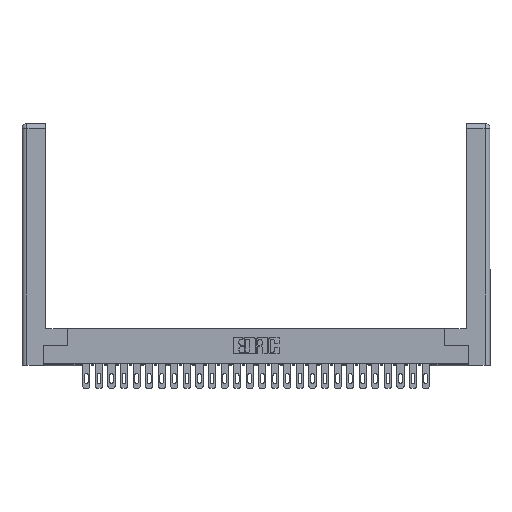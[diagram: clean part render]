
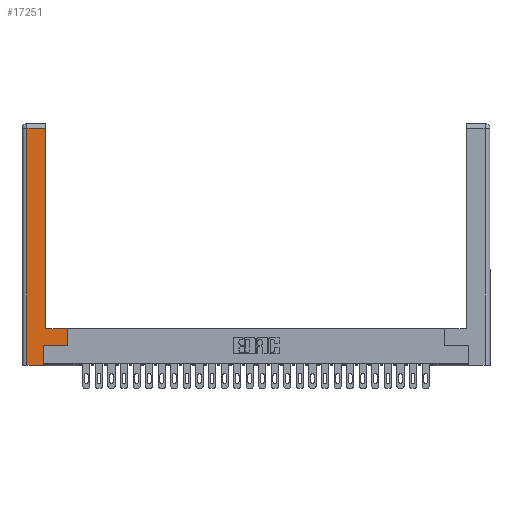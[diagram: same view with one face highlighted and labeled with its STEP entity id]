
A CAD part, top view. The second image highlights one B-rep face of the part: STEP entity #17251.
In plain terms, the highlighted planar face has unit normal (0, 0, 1).
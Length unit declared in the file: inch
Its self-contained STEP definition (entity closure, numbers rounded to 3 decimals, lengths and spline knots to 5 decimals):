
#366 = DIRECTION ( 'NONE',  ( 0., 1., 0. ) ) ;
#792 = VERTEX_POINT ( 'NONE', #11944 ) ;
#869 = LINE ( 'NONE', #4370, #18918 ) ;
#1050 = CARTESIAN_POINT ( 'NONE',  ( 0.265, 0., 0. ) ) ;
#1167 = EDGE_CURVE ( 'NONE', #3997, #29293, #11159, .T. ) ;
#1539 = VERTEX_POINT ( 'NONE', #33579 ) ;
#2278 = CARTESIAN_POINT ( 'NONE',  ( 0.0615, 0., 0. ) ) ;
#3301 = LINE ( 'NONE', #23552, #14991 ) ;
#3997 = VERTEX_POINT ( 'NONE', #1050 ) ;
#4370 = CARTESIAN_POINT ( 'NONE',  ( 0.0615, 2.94, 0. ) ) ;
#4867 = CARTESIAN_POINT ( 'NONE',  ( 0.565, 0.45, 0. ) ) ;
#5165 = VECTOR ( 'NONE', #31440, 39.37008 ) ;
#6160 = CARTESIAN_POINT ( 'NONE',  ( 0.565, 0.245, 0. ) ) ;
#6353 = ORIENTED_EDGE ( 'NONE', *, *, #8636, .T. ) ;
#6360 = VERTEX_POINT ( 'NONE', #4867 ) ;
#8636 = EDGE_CURVE ( 'NONE', #792, #27243, #3301, .T. ) ;
#8668 = EDGE_CURVE ( 'NONE', #28972, #1539, #8693, .T. ) ;
#8693 = LINE ( 'NONE', #2278, #28437 ) ;
#8758 = CARTESIAN_POINT ( 'NONE',  ( 0.265, 0., 0. ) ) ;
#8772 = ORIENTED_EDGE ( 'NONE', *, *, #8668, .T. ) ;
#8880 = DIRECTION ( 'NONE',  ( 1., 0., 0. ) ) ;
#9170 = EDGE_LOOP ( 'NONE', ( #6353, #10185, #8772, #30987, #24147, #32800, #30536, #9584 ) ) ;
#9584 = ORIENTED_EDGE ( 'NONE', *, *, #18812, .T. ) ;
#10185 = ORIENTED_EDGE ( 'NONE', *, *, #20304, .T. ) ;
#10280 = PLANE ( 'NONE',  #26566 ) ;
#10518 = CARTESIAN_POINT ( 'NONE',  ( 0., 0., 0. ) ) ;
#11159 = LINE ( 'NONE', #17291, #24632 ) ;
#11944 = CARTESIAN_POINT ( 'NONE',  ( 0.295, 0.45, 0. ) ) ;
#12806 = VERTEX_POINT ( 'NONE', #29446 ) ;
#13016 = FACE_OUTER_BOUND ( 'NONE', #9170, .T. ) ;
#13491 = VECTOR ( 'NONE', #22264, 39.37008 ) ;
#14577 = CARTESIAN_POINT ( 'NONE',  ( 0.265, 0.245, 0. ) ) ;
#14991 = VECTOR ( 'NONE', #29115, 39.37008 ) ;
#15316 = EDGE_CURVE ( 'NONE', #29293, #12806, #17344, .T. ) ;
#16538 = CARTESIAN_POINT ( 'NONE',  ( 0.295, 2.94, 0. ) ) ;
#17251 = ADVANCED_FACE ( 'NONE', ( #13016 ), #10280, .F. ) ;
#17291 = CARTESIAN_POINT ( 'NONE',  ( 0.265, 0.245, 0. ) ) ;
#17344 = LINE ( 'NONE', #6160, #23263 ) ;
#18119 = CARTESIAN_POINT ( 'NONE',  ( 0.0615, 2.94, 0. ) ) ;
#18812 = EDGE_CURVE ( 'NONE', #6360, #792, #27388, .T. ) ;
#18918 = VECTOR ( 'NONE', #33819, 39.37008 ) ;
#20125 = DIRECTION ( 'NONE',  ( 0., 1., 0. ) ) ;
#20160 = EDGE_CURVE ( 'NONE', #1539, #3997, #24446, .T. ) ;
#20304 = EDGE_CURVE ( 'NONE', #27243, #28972, #869, .T. ) ;
#20725 = CARTESIAN_POINT ( 'NONE',  ( 0.295, 0.45, 0. ) ) ;
#22264 = DIRECTION ( 'NONE',  ( 1., 0., 0. ) ) ;
#23263 = VECTOR ( 'NONE', #8880, 39.37008 ) ;
#23552 = CARTESIAN_POINT ( 'NONE',  ( 0.295, 3., 0. ) ) ;
#23780 = DIRECTION ( 'NONE',  ( 0., -1., 0. ) ) ;
#24147 = ORIENTED_EDGE ( 'NONE', *, *, #1167, .T. ) ;
#24227 = CARTESIAN_POINT ( 'NONE',  ( 0.565, 0.45, 0. ) ) ;
#24446 = LINE ( 'NONE', #8758, #13491 ) ;
#24632 = VECTOR ( 'NONE', #20125, 39.37008 ) ;
#26566 = AXIS2_PLACEMENT_3D ( 'NONE', #10518, #34619, #32057 ) ;
#27243 = VERTEX_POINT ( 'NONE', #16538 ) ;
#27388 = LINE ( 'NONE', #20725, #5165 ) ;
#28437 = VECTOR ( 'NONE', #23780, 39.37008 ) ;
#28770 = LINE ( 'NONE', #24227, #30808 ) ;
#28972 = VERTEX_POINT ( 'NONE', #18119 ) ;
#29115 = DIRECTION ( 'NONE',  ( 0., 1., 0. ) ) ;
#29293 = VERTEX_POINT ( 'NONE', #14577 ) ;
#29446 = CARTESIAN_POINT ( 'NONE',  ( 0.565, 0.245, 0. ) ) ;
#30536 = ORIENTED_EDGE ( 'NONE', *, *, #32088, .T. ) ;
#30808 = VECTOR ( 'NONE', #366, 39.37008 ) ;
#30987 = ORIENTED_EDGE ( 'NONE', *, *, #20160, .T. ) ;
#31440 = DIRECTION ( 'NONE',  ( -1., 0., 0. ) ) ;
#32057 = DIRECTION ( 'NONE',  ( -1., 0., 0. ) ) ;
#32088 = EDGE_CURVE ( 'NONE', #12806, #6360, #28770, .T. ) ;
#32800 = ORIENTED_EDGE ( 'NONE', *, *, #15316, .T. ) ;
#33579 = CARTESIAN_POINT ( 'NONE',  ( 0.0615, 0., 0. ) ) ;
#33819 = DIRECTION ( 'NONE',  ( -1., 0., 0. ) ) ;
#34619 = DIRECTION ( 'NONE',  ( 0., 0., -1. ) ) ;
